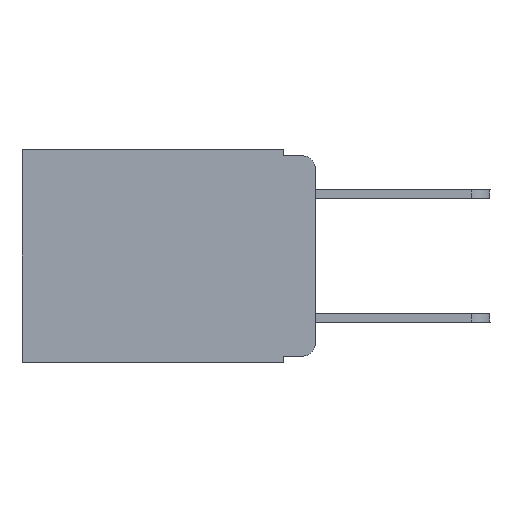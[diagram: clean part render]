
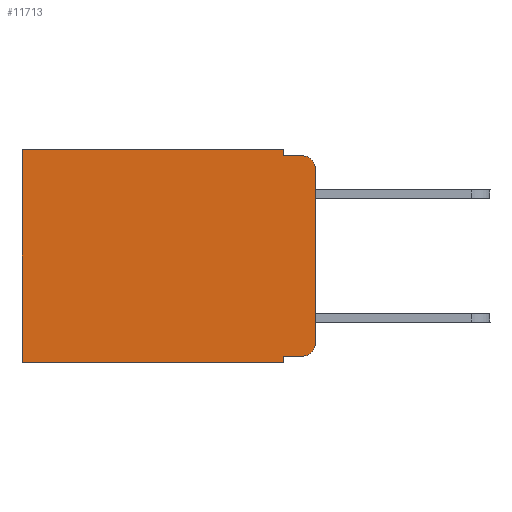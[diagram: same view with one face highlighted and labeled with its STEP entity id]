
A CAD part, left-side view. The second image highlights one B-rep face of the part: STEP entity #11713.
In plain terms, the highlighted planar face has unit normal (-1, 0, 0).
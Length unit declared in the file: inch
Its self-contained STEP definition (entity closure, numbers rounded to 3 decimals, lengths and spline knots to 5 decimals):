
#32 = ORIENTED_EDGE ( 'NONE', *, *, #19678, .F. ) ;
#373 = FACE_OUTER_BOUND ( 'NONE', #2799, .T. ) ;
#621 = EDGE_CURVE ( 'NONE', #13097, #6281, #15870, .T. ) ;
#991 = EDGE_CURVE ( 'NONE', #6281, #6693, #16457, .T. ) ;
#1740 = CARTESIAN_POINT ( 'NONE',  ( 0.298, 0.02, -0.01 ) ) ;
#1913 = VECTOR ( 'NONE', #18705, 39.37008 ) ;
#2012 = CARTESIAN_POINT ( 'NONE',  ( 0.298, 0., 0. ) ) ;
#2082 = VERTEX_POINT ( 'NONE', #18743 ) ;
#2132 = ORIENTED_EDGE ( 'NONE', *, *, #17298, .T. ) ;
#2317 = VERTEX_POINT ( 'NONE', #5536 ) ;
#2318 = EDGE_CURVE ( 'NONE', #2317, #2658, #16485, .T. ) ;
#2374 = LINE ( 'NONE', #14945, #3498 ) ;
#2541 = EDGE_CURVE ( 'NONE', #10604, #6693, #18792, .T. ) ;
#2658 = VERTEX_POINT ( 'NONE', #19309 ) ;
#2799 = EDGE_LOOP ( 'NONE', ( #6258, #13698, #32, #3226, #2132, #7734, #17450, #3533, #11850, #19248 ) ) ;
#2836 = EDGE_CURVE ( 'NONE', #10604, #16141, #8264, .T. ) ;
#3177 = VECTOR ( 'NONE', #4896, 39.37008 ) ;
#3226 = ORIENTED_EDGE ( 'NONE', *, *, #5837, .F. ) ;
#3498 = VECTOR ( 'NONE', #7268, 39.37008 ) ;
#3533 = ORIENTED_EDGE ( 'NONE', *, *, #17259, .F. ) ;
#3776 = VECTOR ( 'NONE', #7069, 39.37008 ) ;
#4017 = VECTOR ( 'NONE', #5640, 39.37008 ) ;
#4272 = DIRECTION ( 'NONE',  ( 0., 0., -1. ) ) ;
#4667 = AXIS2_PLACEMENT_3D ( 'NONE', #13481, #15200, #13870 ) ;
#4896 = DIRECTION ( 'NONE',  ( 0., 0., -1. ) ) ;
#4993 = CARTESIAN_POINT ( 'NONE',  ( 0.298, 0., 0. ) ) ;
#5536 = CARTESIAN_POINT ( 'NONE',  ( 0.298, 0.473, 0. ) ) ;
#5640 = DIRECTION ( 'NONE',  ( 0., -1., 0. ) ) ;
#5828 = DIRECTION ( 'NONE',  ( 0., 0., -1. ) ) ;
#5837 = EDGE_CURVE ( 'NONE', #2082, #17682, #11931, .T. ) ;
#6167 = DIRECTION ( 'NONE',  ( 0., 1., 0. ) ) ;
#6258 = ORIENTED_EDGE ( 'NONE', *, *, #2541, .F. ) ;
#6281 = VERTEX_POINT ( 'NONE', #18541 ) ;
#6488 = VECTOR ( 'NONE', #6167, 39.37008 ) ;
#6503 = DIRECTION ( 'NONE',  ( 0., 0., -1. ) ) ;
#6693 = VERTEX_POINT ( 'NONE', #7351 ) ;
#7069 = DIRECTION ( 'NONE',  ( 0., 0., -1. ) ) ;
#7268 = DIRECTION ( 'NONE',  ( 0., 1., 0. ) ) ;
#7351 = CARTESIAN_POINT ( 'NONE',  ( 0.298, 0., -0.313 ) ) ;
#7734 = ORIENTED_EDGE ( 'NONE', *, *, #2318, .T. ) ;
#8245 = DIRECTION ( 'NONE',  ( 1., 0., 0. ) ) ;
#8257 = DIRECTION ( 'NONE',  ( 0., 0., -1. ) ) ;
#8264 = CIRCLE ( 'NONE', #4667, 0.02 ) ;
#8446 = CARTESIAN_POINT ( 'NONE',  ( 0.298, 0., -0.03 ) ) ;
#10604 = VERTEX_POINT ( 'NONE', #8446 ) ;
#11713 = ADVANCED_FACE ( 'NONE', ( #373 ), #17344, .F. ) ;
#11748 = CARTESIAN_POINT ( 'NONE',  ( 0.298, 0.051, -0.01 ) ) ;
#11850 = ORIENTED_EDGE ( 'NONE', *, *, #621, .T. ) ;
#11931 = LINE ( 'NONE', #14814, #17837 ) ;
#12474 = CARTESIAN_POINT ( 'NONE',  ( 0.298, 0.051, -0.01 ) ) ;
#12717 = CARTESIAN_POINT ( 'NONE',  ( 0.298, 0.051, -0.333 ) ) ;
#12958 = CARTESIAN_POINT ( 'NONE',  ( 0.298, 0.051, -0.343 ) ) ;
#13061 = CARTESIAN_POINT ( 'NONE',  ( 0.298, 0.051, -0.333 ) ) ;
#13097 = VERTEX_POINT ( 'NONE', #13061 ) ;
#13378 = CARTESIAN_POINT ( 'NONE',  ( 0.298, 0.02, -0.313 ) ) ;
#13481 = CARTESIAN_POINT ( 'NONE',  ( 0.298, 0.02, -0.03 ) ) ;
#13698 = ORIENTED_EDGE ( 'NONE', *, *, #2836, .T. ) ;
#13870 = DIRECTION ( 'NONE',  ( 0., 0., -1. ) ) ;
#13950 = LINE ( 'NONE', #17214, #6488 ) ;
#14106 = LINE ( 'NONE', #12474, #1913 ) ;
#14806 = DIRECTION ( 'NONE',  ( -1., 0., 0. ) ) ;
#14814 = CARTESIAN_POINT ( 'NONE',  ( 0.298, 0.051, 0. ) ) ;
#14856 = CARTESIAN_POINT ( 'NONE',  ( 0.298, 0.473, 0. ) ) ;
#14945 = CARTESIAN_POINT ( 'NONE',  ( 0.298, 0., 0. ) ) ;
#15046 = CARTESIAN_POINT ( 'NONE',  ( 0.298, 0.051, 0. ) ) ;
#15144 = LINE ( 'NONE', #15046, #16898 ) ;
#15200 = DIRECTION ( 'NONE',  ( -1., 0., 0. ) ) ;
#15870 = LINE ( 'NONE', #12717, #4017 ) ;
#16123 = AXIS2_PLACEMENT_3D ( 'NONE', #13378, #14806, #8257 ) ;
#16141 = VERTEX_POINT ( 'NONE', #1740 ) ;
#16457 = CIRCLE ( 'NONE', #16123, 0.02 ) ;
#16485 = LINE ( 'NONE', #14856, #3776 ) ;
#16898 = VECTOR ( 'NONE', #5828, 39.37008 ) ;
#17214 = CARTESIAN_POINT ( 'NONE',  ( 0.298, 0., -0.343 ) ) ;
#17259 = EDGE_CURVE ( 'NONE', #13097, #17960, #15144, .T. ) ;
#17298 = EDGE_CURVE ( 'NONE', #2082, #2317, #2374, .T. ) ;
#17323 = AXIS2_PLACEMENT_3D ( 'NONE', #2012, #8245, #6503 ) ;
#17344 = PLANE ( 'NONE',  #17323 ) ;
#17450 = ORIENTED_EDGE ( 'NONE', *, *, #20010, .F. ) ;
#17682 = VERTEX_POINT ( 'NONE', #11748 ) ;
#17837 = VECTOR ( 'NONE', #4272, 39.37008 ) ;
#17960 = VERTEX_POINT ( 'NONE', #12958 ) ;
#18541 = CARTESIAN_POINT ( 'NONE',  ( 0.298, 0.02, -0.333 ) ) ;
#18705 = DIRECTION ( 'NONE',  ( 0., -1., 0. ) ) ;
#18743 = CARTESIAN_POINT ( 'NONE',  ( 0.298, 0.051, 0. ) ) ;
#18792 = LINE ( 'NONE', #4993, #3177 ) ;
#19248 = ORIENTED_EDGE ( 'NONE', *, *, #991, .T. ) ;
#19309 = CARTESIAN_POINT ( 'NONE',  ( 0.298, 0.473, -0.343 ) ) ;
#19678 = EDGE_CURVE ( 'NONE', #17682, #16141, #14106, .T. ) ;
#20010 = EDGE_CURVE ( 'NONE', #17960, #2658, #13950, .T. ) ;
